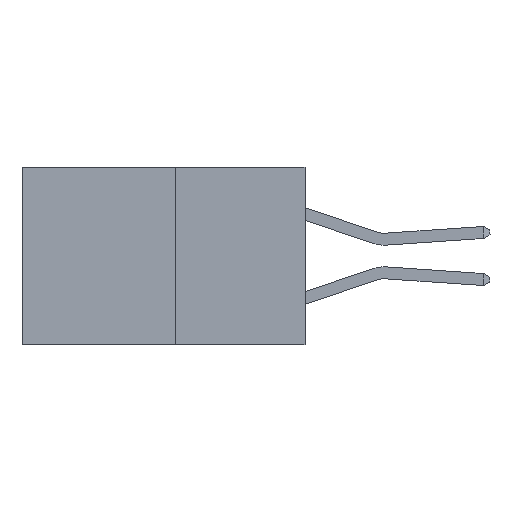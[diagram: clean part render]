
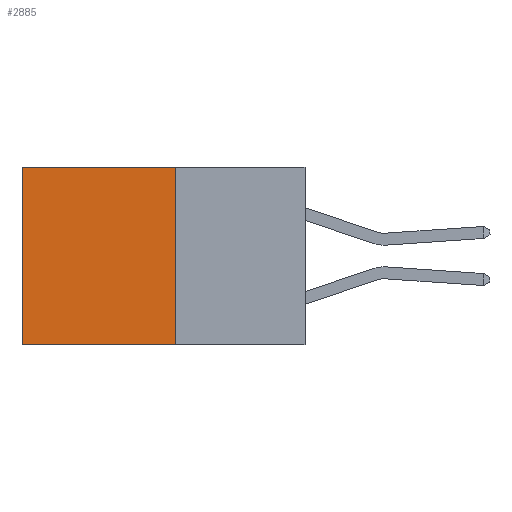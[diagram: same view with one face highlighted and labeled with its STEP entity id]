
A CAD part, left-side view. The second image highlights one B-rep face of the part: STEP entity #2885.
In plain terms, the highlighted planar face has unit normal (-1, 0, 0).
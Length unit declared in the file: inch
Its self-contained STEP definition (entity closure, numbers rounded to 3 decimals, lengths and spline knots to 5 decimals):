
#131 = EDGE_CURVE ( 'NONE', #1442, #4557, #6051, .T. ) ;
#810 = CARTESIAN_POINT ( 'NONE',  ( 0.277, 0.27, -0.37 ) ) ;
#820 = EDGE_CURVE ( 'NONE', #1184, #3226, #8153, .T. ) ;
#849 = DIRECTION ( 'NONE',  ( 1., 0., 0. ) ) ;
#1064 = CARTESIAN_POINT ( 'NONE',  ( 0.277, 0.59, 0. ) ) ;
#1154 = DIRECTION ( 'NONE',  ( 0., 0., -1. ) ) ;
#1184 = VERTEX_POINT ( 'NONE', #4049 ) ;
#1213 = PLANE ( 'NONE',  #5599 ) ;
#1281 = CARTESIAN_POINT ( 'NONE',  ( 0.277, 0.27, 0. ) ) ;
#1442 = VERTEX_POINT ( 'NONE', #1281 ) ;
#1750 = ORIENTED_EDGE ( 'NONE', *, *, #7961, .F. ) ;
#2382 = FACE_OUTER_BOUND ( 'NONE', #8202, .T. ) ;
#2885 = ADVANCED_FACE ( 'NONE', ( #2382 ), #1213, .F. ) ;
#3052 = CARTESIAN_POINT ( 'NONE',  ( 0.277, 0.59, -0.37 ) ) ;
#3226 = VERTEX_POINT ( 'NONE', #7306 ) ;
#3697 = CARTESIAN_POINT ( 'NONE',  ( 0.277, 0.27, -0.37 ) ) ;
#3849 = VECTOR ( 'NONE', #4333, 39.37008 ) ;
#4049 = CARTESIAN_POINT ( 'NONE',  ( 0.277, 0.27, -0.37 ) ) ;
#4264 = CARTESIAN_POINT ( 'NONE',  ( 0.277, 0.27, 0. ) ) ;
#4333 = DIRECTION ( 'NONE',  ( 0., 0., -1. ) ) ;
#4557 = VERTEX_POINT ( 'NONE', #1064 ) ;
#5163 = VECTOR ( 'NONE', #7575, 39.37008 ) ;
#5227 = DIRECTION ( 'NONE',  ( 0., 1., 0. ) ) ;
#5433 = ORIENTED_EDGE ( 'NONE', *, *, #131, .T. ) ;
#5599 = AXIS2_PLACEMENT_3D ( 'NONE', #810, #849, #1154 ) ;
#5600 = ORIENTED_EDGE ( 'NONE', *, *, #8005, .T. ) ;
#5847 = VECTOR ( 'NONE', #5227, 39.37008 ) ;
#5994 = LINE ( 'NONE', #3697, #3849 ) ;
#6051 = LINE ( 'NONE', #4264, #5847 ) ;
#6453 = CARTESIAN_POINT ( 'NONE',  ( 0.277, 0.27, -0.37 ) ) ;
#6868 = ORIENTED_EDGE ( 'NONE', *, *, #820, .F. ) ;
#6905 = LINE ( 'NONE', #3052, #5163 ) ;
#7306 = CARTESIAN_POINT ( 'NONE',  ( 0.277, 0.59, -0.37 ) ) ;
#7575 = DIRECTION ( 'NONE',  ( 0., 0., -1. ) ) ;
#7961 = EDGE_CURVE ( 'NONE', #1442, #1184, #5994, .T. ) ;
#8005 = EDGE_CURVE ( 'NONE', #4557, #3226, #6905, .T. ) ;
#8153 = LINE ( 'NONE', #6453, #8326 ) ;
#8183 = DIRECTION ( 'NONE',  ( 0., 1., 0. ) ) ;
#8202 = EDGE_LOOP ( 'NONE', ( #5600, #6868, #1750, #5433 ) ) ;
#8326 = VECTOR ( 'NONE', #8183, 39.37008 ) ;
